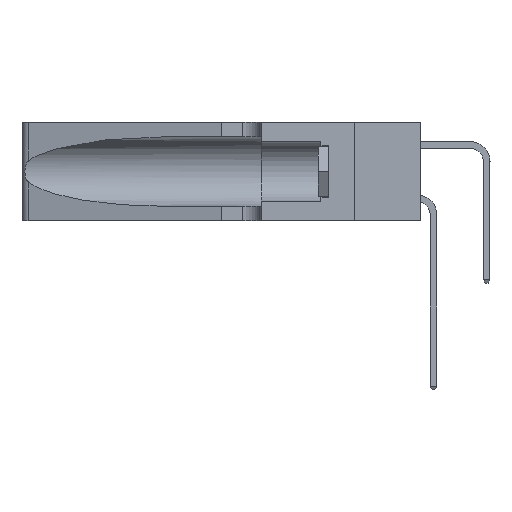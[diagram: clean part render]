
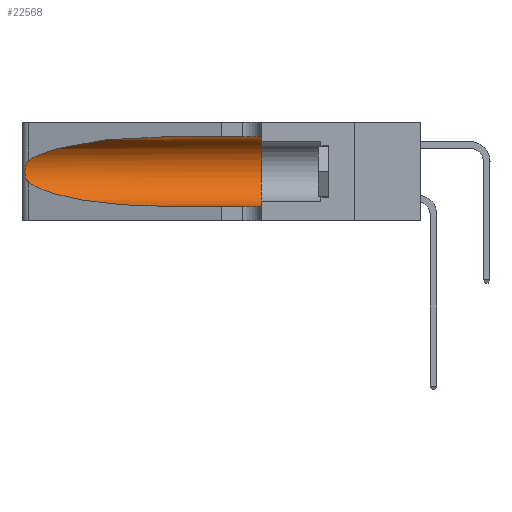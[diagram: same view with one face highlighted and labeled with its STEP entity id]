
A CAD part, left-side view. The second image highlights one B-rep face of the part: STEP entity #22568.
In plain terms, the highlighted cylindrical face has radius 3.308 mm (diameter 6.617 mm), a partial arc.
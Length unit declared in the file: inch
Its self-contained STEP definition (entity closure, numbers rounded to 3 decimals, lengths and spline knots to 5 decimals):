
#1870 = VERTEX_POINT ( 'NONE', #25522 ) ;
#2308 = CARTESIAN_POINT ( 'NONE',  ( 0.18966, 0.96281, 0.05475 ) ) ;
#2479 = DIRECTION ( 'NONE',  ( 0., -1., 0. ) ) ;
#2925 = ORIENTED_EDGE ( 'NONE', *, *, #5398, .T. ) ;
#3901 = DIRECTION ( 'NONE',  ( 0., 0., -1. ) ) ;
#4418 = DIRECTION ( 'NONE',  ( 0., 0., 1. ) ) ;
#5106 = CARTESIAN_POINT ( 'NONE',  ( 0.1305, 0.35, 0.31525 ) ) ;
#5398 = EDGE_CURVE ( 'NONE', #5887, #1870, #28199, .T. ) ;
#5855 = FACE_OUTER_BOUND ( 'NONE', #28449, .T. ) ;
#5887 = VERTEX_POINT ( 'NONE', #18258 ) ;
#6074 = CARTESIAN_POINT ( 'NONE',  ( 0.25487, 1.22718, 0.22369 ) ) ;
#6083 = CARTESIAN_POINT ( 'NONE',  ( 0.1305, 1.61858, 0.31525 ) ) ;
#6570 = VERTEX_POINT ( 'NONE', #15888 ) ;
#6655 = CARTESIAN_POINT ( 'NONE',  ( 0.25789, 1.23486, 0.15765 ) ) ;
#7615 = CARTESIAN_POINT ( 'NONE',  ( 0.26075, 1.23896, 0.178 ) ) ;
#8550 = VERTEX_POINT ( 'NONE', #5106 ) ;
#9259 = VECTOR ( 'NONE', #2479, 39.37008 ) ;
#10317 = CARTESIAN_POINT ( 'NONE',  ( 0.25856, 1.23593, 0.16098 ) ) ;
#10482 = CARTESIAN_POINT ( 'NONE',  ( 0.25555, 1.22994, 0.2215 ) ) ;
#11292 = VECTOR ( 'NONE', #19794, 39.37008 ) ;
#12013 = VERTEX_POINT ( 'NONE', #29938 ) ;
#12074 = DIRECTION ( 'NONE',  ( 0., -1., 0. ) ) ;
#12096 = LINE ( 'NONE', #6083, #11292 ) ;
#12506 = EDGE_CURVE ( 'NONE', #6570, #5887, #16418, .T. ) ;
#13009 = CARTESIAN_POINT ( 'NONE',  ( 0.25639, 1.23184, 0.21858 ) ) ;
#13473 = EDGE_CURVE ( 'NONE', #12013, #32515, #28036, .T. ) ;
#13780 = CARTESIAN_POINT ( 'NONE',  ( 0.25487, 1.22718, 0.14631 ) ) ;
#14149 = CARTESIAN_POINT ( 'NONE',  ( 0.1305, 0.72297, 0.05475 ) ) ;
#15466 = CARTESIAN_POINT ( 'NONE',  ( 0.2373, 1.15595, 0.28018 ) ) ;
#15731 = ORIENTED_EDGE ( 'NONE', *, *, #28885, .F. ) ;
#15888 = CARTESIAN_POINT ( 'NONE',  ( 0.25487, 1.22718, 0.14631 ) ) ;
#16224 = CIRCLE ( 'NONE', #34616, 0.13025 ) ;
#16418 =( BOUNDED_CURVE ( )  B_SPLINE_CURVE ( 3, ( #32890, #32434, #2308, #14149 ),
 .UNSPECIFIED., .F., .F. ) 
 B_SPLINE_CURVE_WITH_KNOTS ( ( 4, 4 ),
 ( 3.44316, 4.71239 ),
 .UNSPECIFIED. ) 
 CURVE ( )  GEOMETRIC_REPRESENTATION_ITEM ( )  RATIONAL_B_SPLINE_CURVE ( ( 1., 0.87, 0.87, 1. ) ) 
 REPRESENTATION_ITEM ( '' )  );
#17985 = CARTESIAN_POINT ( 'NONE',  ( 0.1305, 0.35, 0.185 ) ) ;
#18258 = CARTESIAN_POINT ( 'NONE',  ( 0.1305, 0.72297, 0.05475 ) ) ;
#18303 = CARTESIAN_POINT ( 'NONE',  ( 0.25639, 1.23186, 0.15144 ) ) ;
#19794 = DIRECTION ( 'NONE',  ( 0., -1., 0. ) ) ;
#20713 = ORIENTED_EDGE ( 'NONE', *, *, #12506, .T. ) ;
#21656 = B_SPLINE_CURVE_WITH_KNOTS ( 'NONE', 3,
 ( #23808, #10482, #13009, #35220, #24060, #23927, #32204, #7615, #26831, #10317, #6655, #18303, #35191, #13780 ),
 .UNSPECIFIED., .F., .F.,
 ( 4, 2, 2, 2, 2, 2, 4 ),
 ( 0., 0.00027, 0.00053, 0.00107, 0.0016, 0.00187, 0.00214 ),
 .UNSPECIFIED. ) ;
#22568 = ADVANCED_FACE ( 'NONE', ( #5855 ), #30778, .F. ) ;
#22581 = EDGE_CURVE ( 'NONE', #8550, #1870, #16224, .T. ) ;
#23230 = CARTESIAN_POINT ( 'NONE',  ( 0.1305, 0.72297, 0.31525 ) ) ;
#23808 = CARTESIAN_POINT ( 'NONE',  ( 0.25487, 1.22718, 0.22369 ) ) ;
#23927 = CARTESIAN_POINT ( 'NONE',  ( 0.26018, 1.23835, 0.19895 ) ) ;
#24060 = CARTESIAN_POINT ( 'NONE',  ( 0.25854, 1.2359, 0.20912 ) ) ;
#24104 = CARTESIAN_POINT ( 'NONE',  ( 0.1305, 1.61858, 0.05475 ) ) ;
#25498 = EDGE_CURVE ( 'NONE', #32515, #6570, #21656, .T. ) ;
#25522 = CARTESIAN_POINT ( 'NONE',  ( 0.1305, 0.35, 0.05475 ) ) ;
#25905 = CARTESIAN_POINT ( 'NONE',  ( 0.1305, 1.61858, 0.185 ) ) ;
#26494 = CARTESIAN_POINT ( 'NONE',  ( 0.18966, 0.96281, 0.31525 ) ) ;
#26831 = CARTESIAN_POINT ( 'NONE',  ( 0.26017, 1.23833, 0.17102 ) ) ;
#28036 =( BOUNDED_CURVE ( )  B_SPLINE_CURVE ( 3, ( #23230, #26494, #15466, #29255 ),
 .UNSPECIFIED., .F., .F. ) 
 B_SPLINE_CURVE_WITH_KNOTS ( ( 4, 4 ),
 ( 1.5708, 2.84003 ),
 .UNSPECIFIED. ) 
 CURVE ( )  GEOMETRIC_REPRESENTATION_ITEM ( )  RATIONAL_B_SPLINE_CURVE ( ( 1., 0.87, 0.87, 1. ) ) 
 REPRESENTATION_ITEM ( '' )  );
#28195 = ORIENTED_EDGE ( 'NONE', *, *, #22581, .F. ) ;
#28199 = LINE ( 'NONE', #24104, #9259 ) ;
#28449 = EDGE_LOOP ( 'NONE', ( #28459, #33086, #20713, #2925, #28195, #15731 ) ) ;
#28459 = ORIENTED_EDGE ( 'NONE', *, *, #13473, .T. ) ;
#28773 = DIRECTION ( 'NONE',  ( 0., 1., 0. ) ) ;
#28885 = EDGE_CURVE ( 'NONE', #12013, #8550, #12096, .T. ) ;
#29255 = CARTESIAN_POINT ( 'NONE',  ( 0.25487, 1.22718, 0.22369 ) ) ;
#29938 = CARTESIAN_POINT ( 'NONE',  ( 0.1305, 0.72297, 0.31525 ) ) ;
#30778 = CYLINDRICAL_SURFACE ( 'NONE', #33232, 0.13025 ) ;
#32204 = CARTESIAN_POINT ( 'NONE',  ( 0.26075, 1.23896, 0.19203 ) ) ;
#32434 = CARTESIAN_POINT ( 'NONE',  ( 0.2373, 1.15595, 0.08982 ) ) ;
#32515 = VERTEX_POINT ( 'NONE', #6074 ) ;
#32890 = CARTESIAN_POINT ( 'NONE',  ( 0.25487, 1.22718, 0.14631 ) ) ;
#33086 = ORIENTED_EDGE ( 'NONE', *, *, #25498, .T. ) ;
#33232 = AXIS2_PLACEMENT_3D ( 'NONE', #25905, #12074, #3901 ) ;
#34616 = AXIS2_PLACEMENT_3D ( 'NONE', #17985, #28773, #4418 ) ;
#35191 = CARTESIAN_POINT ( 'NONE',  ( 0.25555, 1.22993, 0.14849 ) ) ;
#35220 = CARTESIAN_POINT ( 'NONE',  ( 0.25787, 1.23484, 0.2124 ) ) ;
